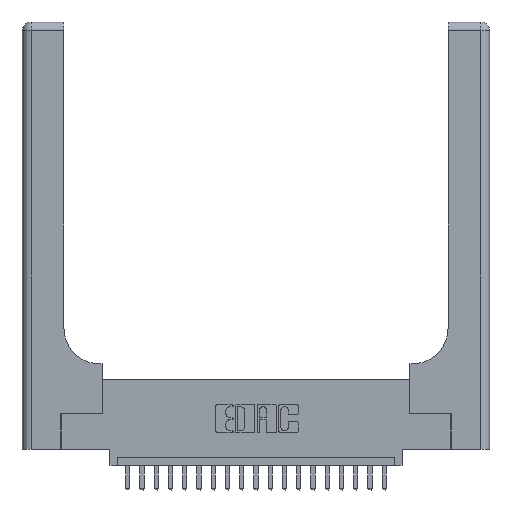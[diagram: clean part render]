
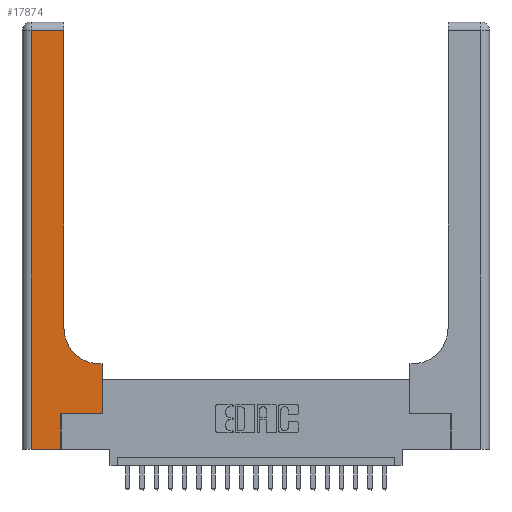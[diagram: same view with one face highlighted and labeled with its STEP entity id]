
A CAD part, top view. The second image highlights one B-rep face of the part: STEP entity #17874.
In plain terms, the highlighted planar face has unit normal (0, 0, 1).
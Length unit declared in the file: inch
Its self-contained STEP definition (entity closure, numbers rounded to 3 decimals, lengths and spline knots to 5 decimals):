
#86 = CARTESIAN_POINT ( 'NONE',  ( 0.06, 2.94, 0.37 ) ) ;
#471 = EDGE_CURVE ( 'NONE', #1093, #15549, #9908, .T. ) ;
#791 = EDGE_CURVE ( 'NONE', #5796, #18494, #2433, .T. ) ;
#1093 = VERTEX_POINT ( 'NONE', #1162 ) ;
#1162 = CARTESIAN_POINT ( 'NONE',  ( 0.06, 0., 0.37 ) ) ;
#1429 = VECTOR ( 'NONE', #8314, 39.37008 ) ;
#1738 = LINE ( 'NONE', #1789, #15027 ) ;
#1789 = CARTESIAN_POINT ( 'NONE',  ( 0.269, 0., 0.37 ) ) ;
#2433 = LINE ( 'NONE', #19279, #7121 ) ;
#2612 = CIRCLE ( 'NONE', #11032, 0.25 ) ;
#2876 = EDGE_CURVE ( 'NONE', #3275, #14372, #8129, .T. ) ;
#2884 = EDGE_CURVE ( 'NONE', #15549, #9964, #1738, .T. ) ;
#2983 = LINE ( 'NONE', #20514, #8229 ) ;
#3275 = VERTEX_POINT ( 'NONE', #21710 ) ;
#3309 = CARTESIAN_POINT ( 'NONE',  ( 0., 3., 0.37 ) ) ;
#3710 = EDGE_CURVE ( 'NONE', #5152, #5796, #2983, .T. ) ;
#4520 = AXIS2_PLACEMENT_3D ( 'NONE', #3309, #12249, #22782 ) ;
#5152 = VERTEX_POINT ( 'NONE', #18080 ) ;
#5416 = DIRECTION ( 'NONE',  ( 0., 1., 0. ) ) ;
#5665 = ORIENTED_EDGE ( 'NONE', *, *, #3710, .T. ) ;
#5693 = ORIENTED_EDGE ( 'NONE', *, *, #19590, .T. ) ;
#5796 = VERTEX_POINT ( 'NONE', #11427 ) ;
#6697 = CARTESIAN_POINT ( 'NONE',  ( 0.269, 0.25, 0.37 ) ) ;
#6815 = ORIENTED_EDGE ( 'NONE', *, *, #18892, .T. ) ;
#6904 = DIRECTION ( 'NONE',  ( -1., 0., 0. ) ) ;
#7121 = VECTOR ( 'NONE', #6904, 39.37008 ) ;
#7360 = CARTESIAN_POINT ( 'NONE',  ( 0.5415, 0.6, 0.37 ) ) ;
#7975 = VECTOR ( 'NONE', #8561, 39.37008 ) ;
#8129 = LINE ( 'NONE', #16784, #15582 ) ;
#8229 = VECTOR ( 'NONE', #17314, 39.37008 ) ;
#8314 = DIRECTION ( 'NONE',  ( 1., 0., 0. ) ) ;
#8491 = CARTESIAN_POINT ( 'NONE',  ( 0., 0., 0.37 ) ) ;
#8561 = DIRECTION ( 'NONE',  ( 1., 0., 0. ) ) ;
#8747 = DIRECTION ( 'NONE',  ( 1., 0., 0. ) ) ;
#9908 = LINE ( 'NONE', #8491, #7975 ) ;
#9964 = VERTEX_POINT ( 'NONE', #12787 ) ;
#10061 = LINE ( 'NONE', #20623, #21265 ) ;
#11032 = AXIS2_PLACEMENT_3D ( 'NONE', #19358, #19289, #8747 ) ;
#11427 = CARTESIAN_POINT ( 'NONE',  ( 0.5585, 0.6, 0.37 ) ) ;
#11687 = EDGE_CURVE ( 'NONE', #15889, #1093, #10061, .T. ) ;
#12249 = DIRECTION ( 'NONE',  ( 0., 0., -1. ) ) ;
#12414 = CARTESIAN_POINT ( 'NONE',  ( 0.269, 0., 0.37 ) ) ;
#12787 = CARTESIAN_POINT ( 'NONE',  ( 0.269, 0.25, 0.37 ) ) ;
#12797 = ORIENTED_EDGE ( 'NONE', *, *, #471, .T. ) ;
#13799 = DIRECTION ( 'NONE',  ( -1., 0., 0. ) ) ;
#14372 = VERTEX_POINT ( 'NONE', #17941 ) ;
#14409 = LINE ( 'NONE', #15418, #15277 ) ;
#14754 = ORIENTED_EDGE ( 'NONE', *, *, #19586, .T. ) ;
#15027 = VECTOR ( 'NONE', #21415, 39.37008 ) ;
#15277 = VECTOR ( 'NONE', #13799, 39.37008 ) ;
#15418 = CARTESIAN_POINT ( 'NONE',  ( 0., 2.94, 0.37 ) ) ;
#15549 = VERTEX_POINT ( 'NONE', #12414 ) ;
#15582 = VECTOR ( 'NONE', #5416, 39.37008 ) ;
#15616 = FACE_OUTER_BOUND ( 'NONE', #18745, .T. ) ;
#15889 = VERTEX_POINT ( 'NONE', #86 ) ;
#16024 = ORIENTED_EDGE ( 'NONE', *, *, #791, .T. ) ;
#16784 = CARTESIAN_POINT ( 'NONE',  ( 0.2915, 3., 0.37 ) ) ;
#16857 = ORIENTED_EDGE ( 'NONE', *, *, #2884, .T. ) ;
#17314 = DIRECTION ( 'NONE',  ( 0., 1., 0. ) ) ;
#17874 = ADVANCED_FACE ( 'NONE', ( #15616 ), #19304, .F. ) ;
#17941 = CARTESIAN_POINT ( 'NONE',  ( 0.2915, 2.94, 0.37 ) ) ;
#18026 = ORIENTED_EDGE ( 'NONE', *, *, #11687, .T. ) ;
#18080 = CARTESIAN_POINT ( 'NONE',  ( 0.5585, 0.25, 0.37 ) ) ;
#18494 = VERTEX_POINT ( 'NONE', #7360 ) ;
#18745 = EDGE_LOOP ( 'NONE', ( #22718, #5693, #18026, #12797, #16857, #14754, #5665, #16024, #6815 ) ) ;
#18892 = EDGE_CURVE ( 'NONE', #18494, #3275, #2612, .T. ) ;
#19063 = LINE ( 'NONE', #6697, #1429 ) ;
#19279 = CARTESIAN_POINT ( 'NONE',  ( 0.2915, 0.6, 0.37 ) ) ;
#19289 = DIRECTION ( 'NONE',  ( 0., 0., -1. ) ) ;
#19304 = PLANE ( 'NONE',  #4520 ) ;
#19358 = CARTESIAN_POINT ( 'NONE',  ( 0.5415, 0.85, 0.37 ) ) ;
#19586 = EDGE_CURVE ( 'NONE', #9964, #5152, #19063, .T. ) ;
#19590 = EDGE_CURVE ( 'NONE', #14372, #15889, #14409, .T. ) ;
#20514 = CARTESIAN_POINT ( 'NONE',  ( 0.5585, 0.25, 0.37 ) ) ;
#20623 = CARTESIAN_POINT ( 'NONE',  ( 0.06, 3., 0.37 ) ) ;
#21265 = VECTOR ( 'NONE', #22431, 39.37008 ) ;
#21415 = DIRECTION ( 'NONE',  ( 0., 1., 0. ) ) ;
#21710 = CARTESIAN_POINT ( 'NONE',  ( 0.2915, 0.85, 0.37 ) ) ;
#22431 = DIRECTION ( 'NONE',  ( 0., -1., 0. ) ) ;
#22718 = ORIENTED_EDGE ( 'NONE', *, *, #2876, .T. ) ;
#22782 = DIRECTION ( 'NONE',  ( -1., 0., 0. ) ) ;
